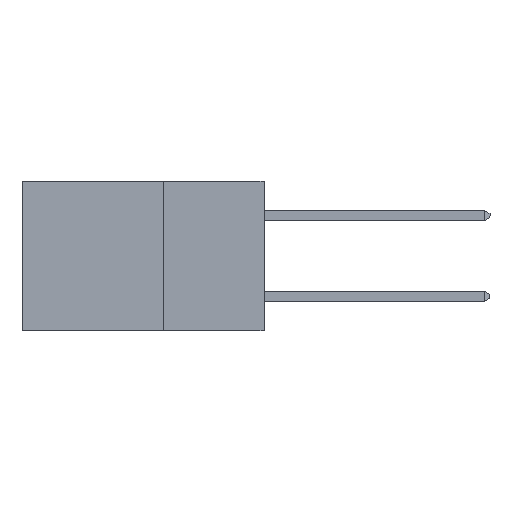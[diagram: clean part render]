
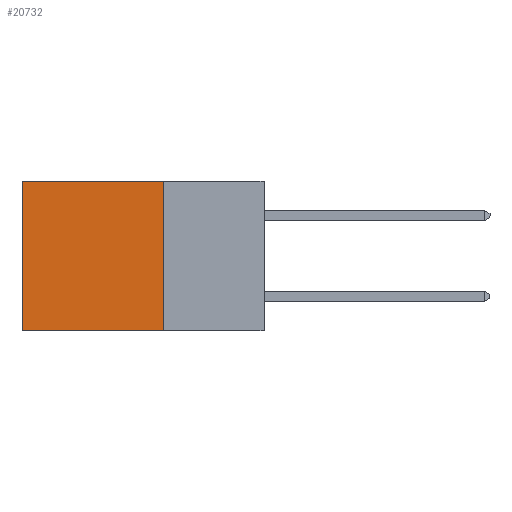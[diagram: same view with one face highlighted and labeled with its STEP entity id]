
A CAD part, left-side view. The second image highlights one B-rep face of the part: STEP entity #20732.
In plain terms, the highlighted planar face has unit normal (-1, 0, 0).
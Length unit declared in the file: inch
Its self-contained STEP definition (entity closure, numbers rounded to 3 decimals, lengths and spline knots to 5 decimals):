
#311 = ORIENTED_EDGE ( 'NONE', *, *, #19947, .F. ) ;
#585 = CARTESIAN_POINT ( 'NONE',  ( 0.298, 0.25, 0. ) ) ;
#650 = VECTOR ( 'NONE', #5199, 39.37008 ) ;
#747 = DIRECTION ( 'NONE',  ( 1., 0., 0. ) ) ;
#1532 = VECTOR ( 'NONE', #14068, 39.37008 ) ;
#3238 = LINE ( 'NONE', #3850, #20479 ) ;
#3850 = CARTESIAN_POINT ( 'NONE',  ( 0.298, 0.25, 0. ) ) ;
#5199 = DIRECTION ( 'NONE',  ( 0., 1., 0. ) ) ;
#5734 = CARTESIAN_POINT ( 'NONE',  ( 0.298, 0.25, 0. ) ) ;
#5976 = LINE ( 'NONE', #585, #1532 ) ;
#6819 = CARTESIAN_POINT ( 'NONE',  ( 0.298, 0.25, -0.37 ) ) ;
#7417 = CARTESIAN_POINT ( 'NONE',  ( 0.298, 0.25, -0.37 ) ) ;
#7852 = VERTEX_POINT ( 'NONE', #17550 ) ;
#8174 = LINE ( 'NONE', #9929, #20466 ) ;
#9561 = LINE ( 'NONE', #6819, #650 ) ;
#9885 = VERTEX_POINT ( 'NONE', #20229 ) ;
#9929 = CARTESIAN_POINT ( 'NONE',  ( 0.298, 0.6, 0. ) ) ;
#10772 = PLANE ( 'NONE',  #17154 ) ;
#11047 = EDGE_CURVE ( 'NONE', #17066, #19353, #9561, .T. ) ;
#11531 = ORIENTED_EDGE ( 'NONE', *, *, #11047, .F. ) ;
#11791 = ORIENTED_EDGE ( 'NONE', *, *, #14861, .T. ) ;
#12461 = DIRECTION ( 'NONE',  ( 0., 0., -1. ) ) ;
#13295 = DIRECTION ( 'NONE',  ( 0., 0., -1. ) ) ;
#14068 = DIRECTION ( 'NONE',  ( 0., 1., 0. ) ) ;
#14861 = EDGE_CURVE ( 'NONE', #7852, #9885, #5976, .T. ) ;
#16736 = ORIENTED_EDGE ( 'NONE', *, *, #18345, .T. ) ;
#17066 = VERTEX_POINT ( 'NONE', #7417 ) ;
#17154 = AXIS2_PLACEMENT_3D ( 'NONE', #5734, #747, #12461 ) ;
#17550 = CARTESIAN_POINT ( 'NONE',  ( 0.298, 0.25, 0. ) ) ;
#17639 = FACE_OUTER_BOUND ( 'NONE', #20171, .T. ) ;
#18345 = EDGE_CURVE ( 'NONE', #9885, #19353, #8174, .T. ) ;
#18956 = DIRECTION ( 'NONE',  ( 0., 0., -1. ) ) ;
#19130 = CARTESIAN_POINT ( 'NONE',  ( 0.298, 0.6, -0.37 ) ) ;
#19353 = VERTEX_POINT ( 'NONE', #19130 ) ;
#19947 = EDGE_CURVE ( 'NONE', #7852, #17066, #3238, .T. ) ;
#20171 = EDGE_LOOP ( 'NONE', ( #16736, #11531, #311, #11791 ) ) ;
#20229 = CARTESIAN_POINT ( 'NONE',  ( 0.298, 0.6, 0. ) ) ;
#20466 = VECTOR ( 'NONE', #13295, 39.37008 ) ;
#20479 = VECTOR ( 'NONE', #18956, 39.37008 ) ;
#20732 = ADVANCED_FACE ( 'NONE', ( #17639 ), #10772, .F. ) ;
